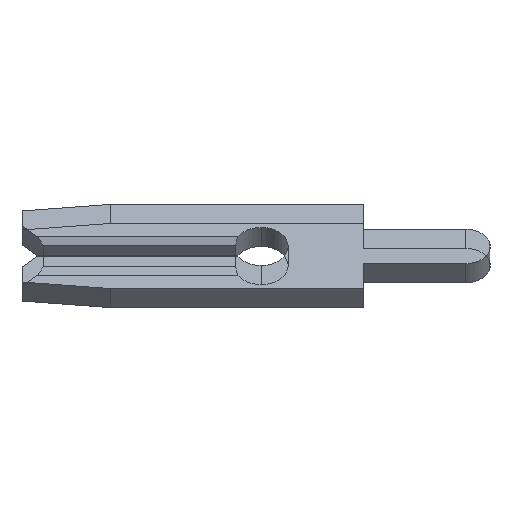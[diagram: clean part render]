
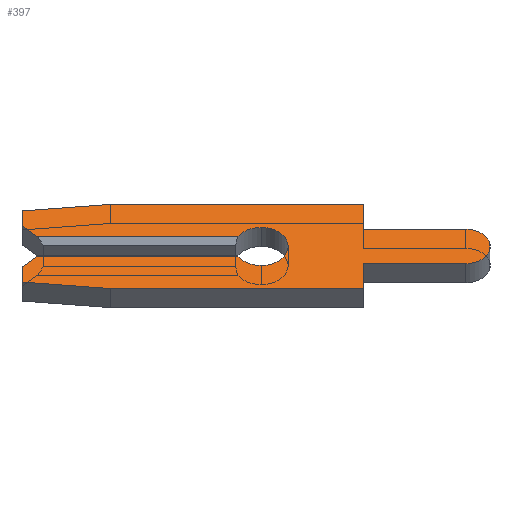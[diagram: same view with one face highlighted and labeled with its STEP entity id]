
A CAD part, left-side view. The second image highlights one B-rep face of the part: STEP entity #397.
In plain terms, the highlighted face is planar.
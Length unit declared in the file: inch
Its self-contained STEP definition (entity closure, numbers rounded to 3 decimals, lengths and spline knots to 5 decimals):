
#5 = CIRCLE ( 'NONE', #2262, 0.026 ) ;
#13 = CARTESIAN_POINT ( 'NONE',  ( -0.013, 0., 0. ) ) ;
#23 = VERTEX_POINT ( 'NONE', #195 ) ;
#33 = LINE ( 'NONE', #2098, #1198 ) ;
#36 = CARTESIAN_POINT ( 'NONE',  ( -0.013, 0., 0.026 ) ) ;
#40 = CARTESIAN_POINT ( 'NONE',  ( -0.013, 0., 0. ) ) ;
#47 = DIRECTION ( 'NONE',  ( 0., 0.995, 0.105 ) ) ;
#49 = VERTEX_POINT ( 'NONE', #1299 ) ;
#104 = VECTOR ( 'NONE', #1072, 39.37008 ) ;
#118 = CARTESIAN_POINT ( 'NONE',  ( -0.013, 0.231, -0.028 ) ) ;
#138 = LINE ( 'NONE', #2724, #1949 ) ;
#176 = CARTESIAN_POINT ( 'NONE',  ( -0.013, 0.02252, 0.013 ) ) ;
#180 = DIRECTION ( 'NONE',  ( 0., 0., -1. ) ) ;
#195 = CARTESIAN_POINT ( 'NONE',  ( -0.013, -0.099, 0.0235 ) ) ;
#200 = VECTOR ( 'NONE', #1896, 39.37008 ) ;
#204 = DIRECTION ( 'NONE',  ( 0., -1., 0. ) ) ;
#208 = ORIENTED_EDGE ( 'NONE', *, *, #1497, .F. ) ;
#227 = VECTOR ( 'NONE', #2204, 39.37008 ) ;
#237 = EDGE_CURVE ( 'NONE', #672, #1857, #2671, .T. ) ;
#298 = EDGE_CURVE ( 'NONE', #796, #1679, #403, .T. ) ;
#300 = FACE_OUTER_BOUND ( 'NONE', #2198, .T. ) ;
#301 = LINE ( 'NONE', #118, #543 ) ;
#334 = CARTESIAN_POINT ( 'NONE',  ( -0.013, 0.216, -0.013 ) ) ;
#337 = EDGE_CURVE ( 'NONE', #1059, #1052, #341, .T. ) ;
#341 = LINE ( 'NONE', #2432, #227 ) ;
#362 = VECTOR ( 'NONE', #921, 39.37008 ) ;
#397 = ADVANCED_FACE ( 'NONE', ( #300 ), #1336, .F. ) ;
#403 = CIRCLE ( 'NONE', #986, 0.0235 ) ;
#411 = EDGE_CURVE ( 'NONE', #1857, #851, #5, .T. ) ;
#417 = CARTESIAN_POINT ( 'NONE',  ( -0.013, -0.099, -0.0235 ) ) ;
#470 = EDGE_CURVE ( 'NONE', #2619, #672, #936, .T. ) ;
#485 = CARTESIAN_POINT ( 'NONE',  ( -0.013, -0.1975, -0.0235 ) ) ;
#524 = ORIENTED_EDGE ( 'NONE', *, *, #237, .F. ) ;
#543 = VECTOR ( 'NONE', #775, 39.37008 ) ;
#550 = ORIENTED_EDGE ( 'NONE', *, *, #2379, .F. ) ;
#551 = CARTESIAN_POINT ( 'NONE',  ( -0.013, 0., -0.026 ) ) ;
#559 = CARTESIAN_POINT ( 'NONE',  ( -0.013, 0., 0. ) ) ;
#576 = DIRECTION ( 'NONE',  ( -1., 0., 0. ) ) ;
#578 = VECTOR ( 'NONE', #2717, 39.37008 ) ;
#624 = DIRECTION ( 'NONE',  ( 0., 0., -1. ) ) ;
#640 = EDGE_CURVE ( 'NONE', #23, #796, #1099, .T. ) ;
#662 = AXIS2_PLACEMENT_3D ( 'NONE', #40, #666, #1942 ) ;
#666 = DIRECTION ( 'NONE',  ( 1., 0., 0. ) ) ;
#672 = VERTEX_POINT ( 'NONE', #334 ) ;
#676 = LINE ( 'NONE', #417, #104 ) ;
#685 = VERTEX_POINT ( 'NONE', #2039 ) ;
#686 = CARTESIAN_POINT ( 'NONE',  ( -0.013, 0.2105, -0.0075 ) ) ;
#760 = CARTESIAN_POINT ( 'NONE',  ( -0.013, -0.099, -0.0235 ) ) ;
#775 = DIRECTION ( 'NONE',  ( 0., 0., 1. ) ) ;
#796 = VERTEX_POINT ( 'NONE', #1430 ) ;
#827 = ORIENTED_EDGE ( 'NONE', *, *, #411, .F. ) ;
#851 = VERTEX_POINT ( 'NONE', #551 ) ;
#852 = EDGE_CURVE ( 'NONE', #1059, #685, #1363, .T. ) ;
#857 = CARTESIAN_POINT ( 'NONE',  ( -0.013, 0.231, -0.04857 ) ) ;
#895 = CARTESIAN_POINT ( 'NONE',  ( -0.013, 0.146, 0.0575 ) ) ;
#901 = AXIS2_PLACEMENT_3D ( 'NONE', #2105, #1865, #180 ) ;
#921 = DIRECTION ( 'NONE',  ( 0., -0.707, 0.707 ) ) ;
#936 = LINE ( 'NONE', #686, #362 ) ;
#986 = AXIS2_PLACEMENT_3D ( 'NONE', #2181, #1771, #1755 ) ;
#993 = VERTEX_POINT ( 'NONE', #1687 ) ;
#994 = VECTOR ( 'NONE', #204, 39.37008 ) ;
#1003 = CARTESIAN_POINT ( 'NONE',  ( -0.013, -0.099, 0.0235 ) ) ;
#1020 = DIRECTION ( 'NONE',  ( 0., -1., 0. ) ) ;
#1023 = ORIENTED_EDGE ( 'NONE', *, *, #2538, .F. ) ;
#1036 = CARTESIAN_POINT ( 'NONE',  ( -0.013, 0.146, -0.0575 ) ) ;
#1038 = VERTEX_POINT ( 'NONE', #1274 ) ;
#1052 = VERTEX_POINT ( 'NONE', #176 ) ;
#1057 = CARTESIAN_POINT ( 'NONE',  ( -0.013, 0., -0.013 ) ) ;
#1059 = VERTEX_POINT ( 'NONE', #1887 ) ;
#1060 = VECTOR ( 'NONE', #1020, 39.37008 ) ;
#1072 = DIRECTION ( 'NONE',  ( 0., 1., 0. ) ) ;
#1091 = DIRECTION ( 'NONE',  ( 0., 0., 1. ) ) ;
#1099 = LINE ( 'NONE', #1003, #1060 ) ;
#1142 = CARTESIAN_POINT ( 'NONE',  ( -0.013, 0.231, 0.04857 ) ) ;
#1148 = EDGE_CURVE ( 'NONE', #1802, #1052, #1561, .T. ) ;
#1198 = VECTOR ( 'NONE', #1691, 39.37008 ) ;
#1199 = EDGE_CURVE ( 'NONE', #2579, #993, #2363, .T. ) ;
#1234 = CARTESIAN_POINT ( 'NONE',  ( -0.013, 0.2105, 0.0075 ) ) ;
#1274 = CARTESIAN_POINT ( 'NONE',  ( -0.013, 0.231, -0.04857 ) ) ;
#1281 = EDGE_CURVE ( 'NONE', #1777, #1817, #33, .T. ) ;
#1299 = CARTESIAN_POINT ( 'NONE',  ( -0.013, -0.099, 0.0575 ) ) ;
#1336 = PLANE ( 'NONE',  #662 ) ;
#1353 = CARTESIAN_POINT ( 'NONE',  ( -0.013, 0.146, 0.0575 ) ) ;
#1363 = LINE ( 'NONE', #1234, #578 ) ;
#1374 = EDGE_CURVE ( 'NONE', #685, #1777, #1599, .T. ) ;
#1424 = LINE ( 'NONE', #1784, #2200 ) ;
#1430 = CARTESIAN_POINT ( 'NONE',  ( -0.013, -0.1975, 0.0235 ) ) ;
#1497 = EDGE_CURVE ( 'NONE', #851, #1802, #1903, .T. ) ;
#1511 = CARTESIAN_POINT ( 'NONE',  ( -0.013, -0.099, -0.0575 ) ) ;
#1513 = DIRECTION ( 'NONE',  ( 0., -1., 0. ) ) ;
#1522 = DIRECTION ( 'NONE',  ( -1., 0., 0. ) ) ;
#1544 = DIRECTION ( 'NONE',  ( 0., 0., -1. ) ) ;
#1561 = CIRCLE ( 'NONE', #901, 0.026 ) ;
#1599 = LINE ( 'NONE', #1662, #2057 ) ;
#1645 = EDGE_CURVE ( 'NONE', #993, #1038, #2303, .T. ) ;
#1662 = CARTESIAN_POINT ( 'NONE',  ( -0.013, 0.231, 0.028 ) ) ;
#1679 = VERTEX_POINT ( 'NONE', #485 ) ;
#1687 = CARTESIAN_POINT ( 'NONE',  ( -0.013, 0.146, -0.0575 ) ) ;
#1691 = DIRECTION ( 'NONE',  ( 0., -0.995, 0.105 ) ) ;
#1695 = VECTOR ( 'NONE', #47, 39.37008 ) ;
#1702 = ORIENTED_EDGE ( 'NONE', *, *, #470, .F. ) ;
#1727 = ORIENTED_EDGE ( 'NONE', *, *, #1374, .F. ) ;
#1752 = AXIS2_PLACEMENT_3D ( 'NONE', #13, #1522, #624 ) ;
#1755 = DIRECTION ( 'NONE',  ( 0., 0., 1. ) ) ;
#1771 = DIRECTION ( 'NONE',  ( 1., 0., 0. ) ) ;
#1777 = VERTEX_POINT ( 'NONE', #1142 ) ;
#1784 = CARTESIAN_POINT ( 'NONE',  ( -0.013, -0.099, 0.0575 ) ) ;
#1802 = VERTEX_POINT ( 'NONE', #36 ) ;
#1817 = VERTEX_POINT ( 'NONE', #1353 ) ;
#1857 = VERTEX_POINT ( 'NONE', #1968 ) ;
#1865 = DIRECTION ( 'NONE',  ( -1., 0., 0. ) ) ;
#1886 = ORIENTED_EDGE ( 'NONE', *, *, #2328, .F. ) ;
#1887 = CARTESIAN_POINT ( 'NONE',  ( -0.013, 0.216, 0.013 ) ) ;
#1896 = DIRECTION ( 'NONE',  ( 0., 1., 0. ) ) ;
#1903 = CIRCLE ( 'NONE', #1752, 0.026 ) ;
#1942 = DIRECTION ( 'NONE',  ( 0., 0., -1. ) ) ;
#1949 = VECTOR ( 'NONE', #2145, 39.37008 ) ;
#1953 = VECTOR ( 'NONE', #1513, 39.37008 ) ;
#1962 = ORIENTED_EDGE ( 'NONE', *, *, #1281, .F. ) ;
#1968 = CARTESIAN_POINT ( 'NONE',  ( -0.013, 0.02252, -0.013 ) ) ;
#1990 = ORIENTED_EDGE ( 'NONE', *, *, #2237, .F. ) ;
#2039 = CARTESIAN_POINT ( 'NONE',  ( -0.013, 0.231, 0.028 ) ) ;
#2057 = VECTOR ( 'NONE', #1091, 39.37008 ) ;
#2098 = CARTESIAN_POINT ( 'NONE',  ( -0.013, 0.231, 0.04857 ) ) ;
#2105 = CARTESIAN_POINT ( 'NONE',  ( -0.013, 0., 0. ) ) ;
#2125 = VERTEX_POINT ( 'NONE', #760 ) ;
#2126 = ORIENTED_EDGE ( 'NONE', *, *, #852, .F. ) ;
#2145 = DIRECTION ( 'NONE',  ( 0., 0., -1. ) ) ;
#2181 = CARTESIAN_POINT ( 'NONE',  ( -0.013, -0.1975, 0. ) ) ;
#2198 = EDGE_LOOP ( 'NONE', ( #2239, #2737, #208, #827, #524, #1702, #1990, #2707, #2429, #1886, #1023, #2537, #2708, #2552, #550, #1962, #1727, #2126 ) ) ;
#2200 = VECTOR ( 'NONE', #1544, 39.37008 ) ;
#2204 = DIRECTION ( 'NONE',  ( 0., -1., 0. ) ) ;
#2237 = EDGE_CURVE ( 'NONE', #1038, #2619, #301, .T. ) ;
#2239 = ORIENTED_EDGE ( 'NONE', *, *, #337, .T. ) ;
#2262 = AXIS2_PLACEMENT_3D ( 'NONE', #559, #576, #2744 ) ;
#2271 = LINE ( 'NONE', #895, #994 ) ;
#2303 = LINE ( 'NONE', #857, #1695 ) ;
#2328 = EDGE_CURVE ( 'NONE', #2125, #2579, #138, .T. ) ;
#2363 = LINE ( 'NONE', #1036, #200 ) ;
#2379 = EDGE_CURVE ( 'NONE', #1817, #49, #2271, .T. ) ;
#2394 = EDGE_CURVE ( 'NONE', #49, #23, #1424, .T. ) ;
#2429 = ORIENTED_EDGE ( 'NONE', *, *, #1199, .F. ) ;
#2432 = CARTESIAN_POINT ( 'NONE',  ( -0.013, 0.231, 0.013 ) ) ;
#2537 = ORIENTED_EDGE ( 'NONE', *, *, #298, .F. ) ;
#2538 = EDGE_CURVE ( 'NONE', #1679, #2125, #676, .T. ) ;
#2552 = ORIENTED_EDGE ( 'NONE', *, *, #2394, .F. ) ;
#2579 = VERTEX_POINT ( 'NONE', #1511 ) ;
#2610 = CARTESIAN_POINT ( 'NONE',  ( -0.013, 0.231, -0.028 ) ) ;
#2619 = VERTEX_POINT ( 'NONE', #2610 ) ;
#2671 = LINE ( 'NONE', #1057, #1953 ) ;
#2707 = ORIENTED_EDGE ( 'NONE', *, *, #1645, .F. ) ;
#2708 = ORIENTED_EDGE ( 'NONE', *, *, #640, .F. ) ;
#2717 = DIRECTION ( 'NONE',  ( 0., 0.707, 0.707 ) ) ;
#2724 = CARTESIAN_POINT ( 'NONE',  ( -0.013, -0.099, -0.0575 ) ) ;
#2737 = ORIENTED_EDGE ( 'NONE', *, *, #1148, .F. ) ;
#2744 = DIRECTION ( 'NONE',  ( 0., 0., -1. ) ) ;
